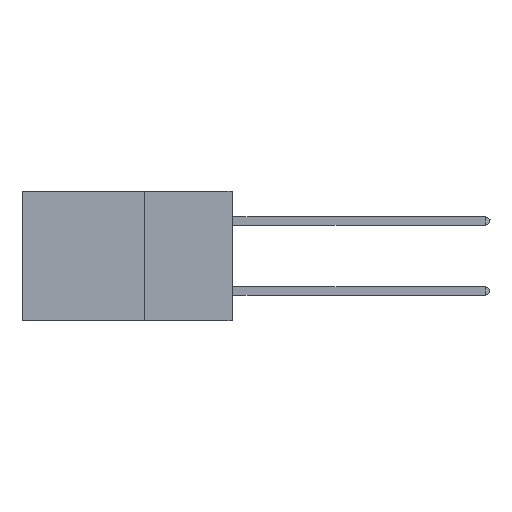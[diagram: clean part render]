
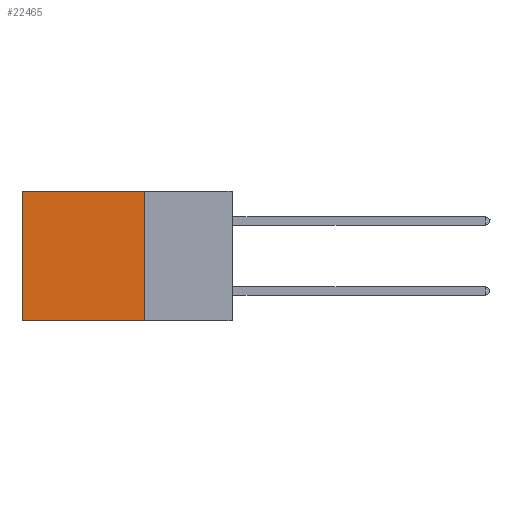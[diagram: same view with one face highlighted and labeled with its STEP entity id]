
A CAD part, left-side view. The second image highlights one B-rep face of the part: STEP entity #22465.
In plain terms, the highlighted planar face has unit normal (-1, 0, 0).
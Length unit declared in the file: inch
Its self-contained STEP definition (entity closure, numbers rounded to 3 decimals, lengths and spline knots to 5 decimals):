
#789 = EDGE_CURVE ( 'NONE', #6724, #4915, #18398, .T. ) ;
#864 = ORIENTED_EDGE ( 'NONE', *, *, #1592, .F. ) ;
#1234 = DIRECTION ( 'NONE',  ( 0., 0., -1. ) ) ;
#1592 = EDGE_CURVE ( 'NONE', #22855, #6724, #5133, .T. ) ;
#1698 = CARTESIAN_POINT ( 'NONE',  ( 0.2875, 0.25, 0. ) ) ;
#2375 = DIRECTION ( 'NONE',  ( 0., 0., -1. ) ) ;
#2787 = LINE ( 'NONE', #4680, #23087 ) ;
#3428 = ORIENTED_EDGE ( 'NONE', *, *, #8819, .T. ) ;
#3569 = DIRECTION ( 'NONE',  ( 0., 1., 0. ) ) ;
#3645 = CARTESIAN_POINT ( 'NONE',  ( 0.2875, 0.25, 0. ) ) ;
#3922 = DIRECTION ( 'NONE',  ( 1., 0., 0. ) ) ;
#4680 = CARTESIAN_POINT ( 'NONE',  ( 0.2875, 0.6, 0. ) ) ;
#4915 = VERTEX_POINT ( 'NONE', #21728 ) ;
#5133 = LINE ( 'NONE', #1698, #18535 ) ;
#5177 = LINE ( 'NONE', #3645, #6238 ) ;
#5346 = CARTESIAN_POINT ( 'NONE',  ( 0.2875, 0.25, -0.37 ) ) ;
#6238 = VECTOR ( 'NONE', #8982, 39.37008 ) ;
#6724 = VERTEX_POINT ( 'NONE', #13610 ) ;
#6959 = CARTESIAN_POINT ( 'NONE',  ( 0.2875, 0.6, 0. ) ) ;
#7281 = EDGE_CURVE ( 'NONE', #15908, #4915, #2787, .T. ) ;
#8819 = EDGE_CURVE ( 'NONE', #22855, #15908, #5177, .T. ) ;
#8982 = DIRECTION ( 'NONE',  ( 0., 1., 0. ) ) ;
#9812 = ORIENTED_EDGE ( 'NONE', *, *, #789, .F. ) ;
#11040 = FACE_OUTER_BOUND ( 'NONE', #13850, .T. ) ;
#11271 = PLANE ( 'NONE',  #21119 ) ;
#13610 = CARTESIAN_POINT ( 'NONE',  ( 0.2875, 0.25, -0.37 ) ) ;
#13850 = EDGE_LOOP ( 'NONE', ( #22890, #9812, #864, #3428 ) ) ;
#15908 = VERTEX_POINT ( 'NONE', #6959 ) ;
#16573 = CARTESIAN_POINT ( 'NONE',  ( 0.2875, 0.25, 0. ) ) ;
#18398 = LINE ( 'NONE', #5346, #21155 ) ;
#18535 = VECTOR ( 'NONE', #1234, 39.37008 ) ;
#20182 = CARTESIAN_POINT ( 'NONE',  ( 0.2875, 0.25, 0. ) ) ;
#21119 = AXIS2_PLACEMENT_3D ( 'NONE', #20182, #3922, #2375 ) ;
#21155 = VECTOR ( 'NONE', #3569, 39.37008 ) ;
#21728 = CARTESIAN_POINT ( 'NONE',  ( 0.2875, 0.6, -0.37 ) ) ;
#22465 = ADVANCED_FACE ( 'NONE', ( #11040 ), #11271, .F. ) ;
#22618 = DIRECTION ( 'NONE',  ( 0., 0., -1. ) ) ;
#22855 = VERTEX_POINT ( 'NONE', #16573 ) ;
#22890 = ORIENTED_EDGE ( 'NONE', *, *, #7281, .T. ) ;
#23087 = VECTOR ( 'NONE', #22618, 39.37008 ) ;
